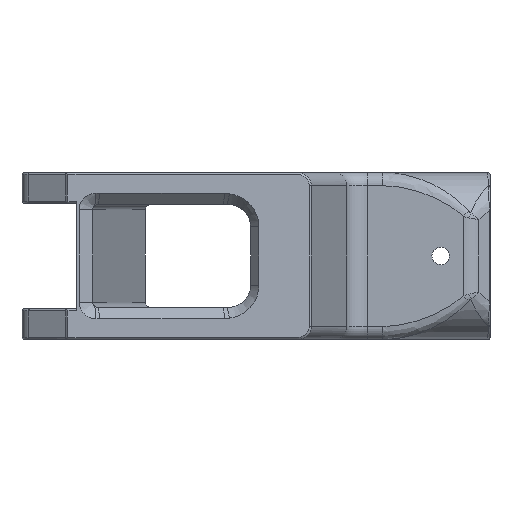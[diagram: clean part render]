
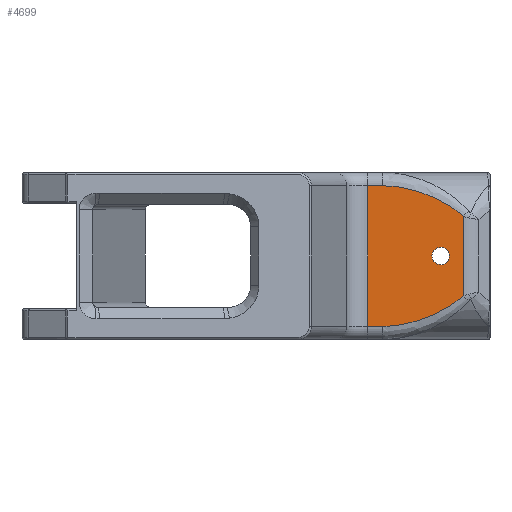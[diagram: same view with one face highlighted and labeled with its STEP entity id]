
A CAD part, front view. The second image highlights one B-rep face of the part: STEP entity #4699.
In plain terms, the highlighted planar face has unit normal (0, -1, 0).
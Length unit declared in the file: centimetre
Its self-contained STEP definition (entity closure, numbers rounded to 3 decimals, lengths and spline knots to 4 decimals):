
#85=FACE_BOUND($,#801,.T.);
#157=CIRCLE($,#5006,0.2);
#343=PLANE($,#5005);
#501=FACE_OUTER_BOUND($,#800,.T.);
#800=EDGE_LOOP($,(#3593,#3594,#3595,#3596,#3597,#3598));
#801=EDGE_LOOP($,(#3599));
#1174=LINE($,#8336,#1566);
#1175=LINE($,#8347,#1567);
#1176=LINE($,#8349,#1568);
#1177=LINE($,#8351,#1569);
#1566=VECTOR($,#5647,1.8036);
#1567=VECTOR($,#5650,0.3447);
#1568=VECTOR($,#5651,3.2);
#1569=VECTOR($,#5652,0.3447);
#1899=B_SPLINE_CURVE_WITH_KNOTS($,3,(#8339,#8340,#8341,#8342,#8343,#8344,
#8345),.UNSPECIFIED.,.F.,.F.,(4,1,1,1,4),(0.,0.5714,
1.1428,1.7141,1.9998),.UNSPECIFIED.);
#1900=B_SPLINE_CURVE_WITH_KNOTS($,3,(#8352,#8353,#8354,#8355,#8356,#8357,
#8358),.UNSPECIFIED.,.F.,.F.,(4,1,1,1,4),(3.8425,4.1282,
4.6996,5.271,5.8424),.UNSPECIFIED.);
#2183=VERTEX_POINT($,#8243);
#2185=VERTEX_POINT($,#8298);
#2186=VERTEX_POINT($,#8338);
#2187=VERTEX_POINT($,#8346);
#2188=VERTEX_POINT($,#8348);
#2189=VERTEX_POINT($,#8350);
#2190=VERTEX_POINT($,#8359);
#2711=EDGE_CURVE($,#2185,#2183,#1174,.T.);
#2712=EDGE_CURVE($,#2186,#2185,#1899,.T.);
#2713=EDGE_CURVE($,#2187,#2186,#1175,.T.);
#2714=EDGE_CURVE($,#2187,#2188,#1176,.T.);
#2715=EDGE_CURVE($,#2189,#2188,#1177,.T.);
#2716=EDGE_CURVE($,#2183,#2189,#1900,.T.);
#2717=EDGE_CURVE($,#2190,#2190,#157,.T.);
#3593=ORIENTED_EDGE($,*,*,#2711,.F.);
#3594=ORIENTED_EDGE($,*,*,#2712,.F.);
#3595=ORIENTED_EDGE($,*,*,#2713,.F.);
#3596=ORIENTED_EDGE($,*,*,#2714,.T.);
#3597=ORIENTED_EDGE($,*,*,#2715,.F.);
#3598=ORIENTED_EDGE($,*,*,#2716,.F.);
#3599=ORIENTED_EDGE($,*,*,#2717,.F.);
#4699=ADVANCED_FACE($,(#501,#85),#343,.T.);
#5005=AXIS2_PLACEMENT_3D($,#8337,#5648,#5649);
#5006=AXIS2_PLACEMENT_3D($,#8360,#5653,#5654);
#5647=DIRECTION($,(0.,0.,-1.));
#5648=DIRECTION('center_axis',(0.,-1.,0.));
#5649=DIRECTION('ref_axis',(0.,0.,-1.));
#5650=DIRECTION($,(1.,0.,0.));
#5651=DIRECTION($,(0.,0.,-1.));
#5652=DIRECTION($,(-1.,0.,0.));
#5653=DIRECTION('center_axis',(0.,-1.,0.));
#5654=DIRECTION('ref_axis',(1.,0.,0.));
#8243=CARTESIAN_POINT('',(0.5606,-2.5877,-20.8018));
#8298=CARTESIAN_POINT('',(0.5606,-2.5877,-18.9982));
#8336=CARTESIAN_POINT($,(0.5606,-2.5877,-19.8897));
#8337=CARTESIAN_POINT('Origin',(0.6464,-2.5877,-19.9));
#8338=CARTESIAN_POINT('',(-1.2702,-2.5877,-18.3));
#8339=CARTESIAN_POINT('Ctrl Pts',(-1.2702,-2.5877,-18.3));
#8340=CARTESIAN_POINT('Ctrl Pts',(-1.0797,-2.5877,-18.3));
#8341=CARTESIAN_POINT('Ctrl Pts',(-0.6992,-2.5877,
-18.3476));
#8342=CARTESIAN_POINT('Ctrl Pts',(-0.1559,-2.5877,
-18.5305));
#8343=CARTESIAN_POINT('Ctrl Pts',(0.2634,-2.5877,-18.7585));
#8344=CARTESIAN_POINT('Ctrl Pts',(0.4905,-2.5877,-18.9339));
#8345=CARTESIAN_POINT('Ctrl Pts',(0.5606,-2.5877,-18.9982));
#8346=CARTESIAN_POINT('',(-1.6149,-2.5877,-18.3));
#8347=CARTESIAN_POINT($,(-1.9118,-2.5877,-18.3));
#8348=CARTESIAN_POINT('',(-1.6149,-2.5877,-21.5));
#8349=CARTESIAN_POINT($,(-1.6149,-2.5877,-19.9));
#8350=CARTESIAN_POINT('',(-1.2702,-2.5877,-21.5));
#8351=CARTESIAN_POINT($,(-1.9118,-2.5877,-21.5));
#8352=CARTESIAN_POINT('Ctrl Pts',(0.5606,-2.5877,-20.8018));
#8353=CARTESIAN_POINT('Ctrl Pts',(0.4905,-2.5877,-20.8661));
#8354=CARTESIAN_POINT('Ctrl Pts',(0.2634,-2.5877,-21.0415));
#8355=CARTESIAN_POINT('Ctrl Pts',(-0.1559,-2.5877,
-21.2695));
#8356=CARTESIAN_POINT('Ctrl Pts',(-0.6992,-2.5877,
-21.4524));
#8357=CARTESIAN_POINT('Ctrl Pts',(-1.0797,-2.5877,-21.5));
#8358=CARTESIAN_POINT('Ctrl Pts',(-1.2702,-2.5877,-21.5));
#8359=CARTESIAN_POINT('',(-0.1536,-2.5877,-19.9));
#8360=CARTESIAN_POINT('Origin',(0.0464,-2.5877,-19.9));
